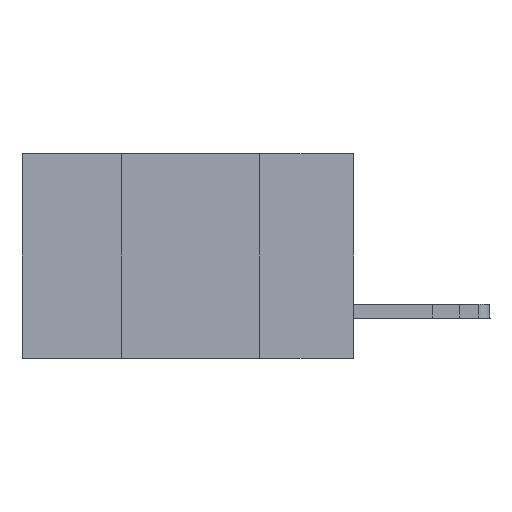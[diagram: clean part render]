
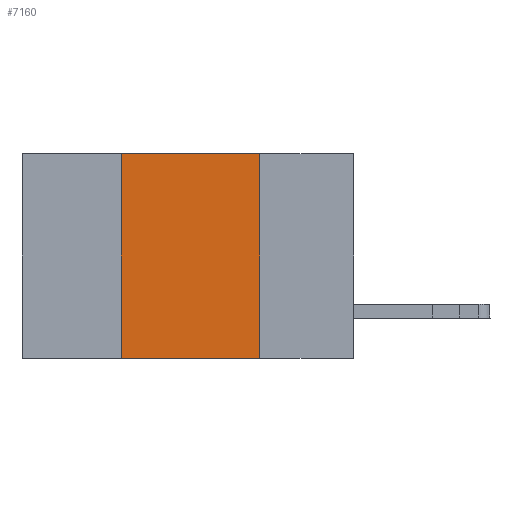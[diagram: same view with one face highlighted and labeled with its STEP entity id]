
A CAD part, left-side view. The second image highlights one B-rep face of the part: STEP entity #7160.
In plain terms, the highlighted planar face has unit normal (-1, 0, 0).
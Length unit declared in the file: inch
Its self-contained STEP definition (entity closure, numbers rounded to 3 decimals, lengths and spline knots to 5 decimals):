
#459 = CARTESIAN_POINT ( 'NONE',  ( 0., 0.17, 0. ) ) ;
#1146 = CARTESIAN_POINT ( 'NONE',  ( 0., 0.42, 0. ) ) ;
#1173 = ORIENTED_EDGE ( 'NONE', *, *, #10435, .F. ) ;
#1209 = DIRECTION ( 'NONE',  ( 0., 0., 1. ) ) ;
#1407 = CARTESIAN_POINT ( 'NONE',  ( 0., 0.42, 0. ) ) ;
#1849 = CARTESIAN_POINT ( 'NONE',  ( 0., 0.42, -0.37 ) ) ;
#2110 = LINE ( 'NONE', #5864, #5175 ) ;
#2171 = LINE ( 'NONE', #1146, #14500 ) ;
#2188 = ORIENTED_EDGE ( 'NONE', *, *, #4764, .F. ) ;
#3133 = VERTEX_POINT ( 'NONE', #7267 ) ;
#3435 = CARTESIAN_POINT ( 'NONE',  ( 0., 0.6, 0. ) ) ;
#3491 = DIRECTION ( 'NONE',  ( 0., 0., -1. ) ) ;
#3569 = CARTESIAN_POINT ( 'NONE',  ( 0., 0.6, 0. ) ) ;
#4626 = VECTOR ( 'NONE', #13053, 39.37008 ) ;
#4764 = EDGE_CURVE ( 'NONE', #15039, #12694, #2171, .T. ) ;
#4855 = CARTESIAN_POINT ( 'NONE',  ( 0., 0.6, -0.37 ) ) ;
#5175 = VECTOR ( 'NONE', #7088, 39.37008 ) ;
#5864 = CARTESIAN_POINT ( 'NONE',  ( 0., 0.17, 0. ) ) ;
#6763 = LINE ( 'NONE', #3569, #9524 ) ;
#7088 = DIRECTION ( 'NONE',  ( 0., 0., -1. ) ) ;
#7160 = ADVANCED_FACE ( 'NONE', ( #15519 ), #15268, .F. ) ;
#7267 = CARTESIAN_POINT ( 'NONE',  ( 0., 0.17, -0.37 ) ) ;
#8029 = ORIENTED_EDGE ( 'NONE', *, *, #12510, .F. ) ;
#9524 = VECTOR ( 'NONE', #10814, 39.37008 ) ;
#10435 = EDGE_CURVE ( 'NONE', #12898, #3133, #2110, .T. ) ;
#10563 = AXIS2_PLACEMENT_3D ( 'NONE', #3435, #10737, #3491 ) ;
#10591 = LINE ( 'NONE', #4855, #4626 ) ;
#10737 = DIRECTION ( 'NONE',  ( 1., 0., 0. ) ) ;
#10814 = DIRECTION ( 'NONE',  ( 0., -1., 0. ) ) ;
#12510 = EDGE_CURVE ( 'NONE', #12694, #12898, #6763, .T. ) ;
#12694 = VERTEX_POINT ( 'NONE', #1407 ) ;
#12898 = VERTEX_POINT ( 'NONE', #459 ) ;
#13053 = DIRECTION ( 'NONE',  ( 0., -1., 0. ) ) ;
#13584 = EDGE_LOOP ( 'NONE', ( #1173, #8029, #2188, #13781 ) ) ;
#13683 = EDGE_CURVE ( 'NONE', #15039, #3133, #10591, .T. ) ;
#13781 = ORIENTED_EDGE ( 'NONE', *, *, #13683, .T. ) ;
#14500 = VECTOR ( 'NONE', #1209, 39.37008 ) ;
#15039 = VERTEX_POINT ( 'NONE', #1849 ) ;
#15268 = PLANE ( 'NONE',  #10563 ) ;
#15519 = FACE_OUTER_BOUND ( 'NONE', #13584, .T. ) ;
